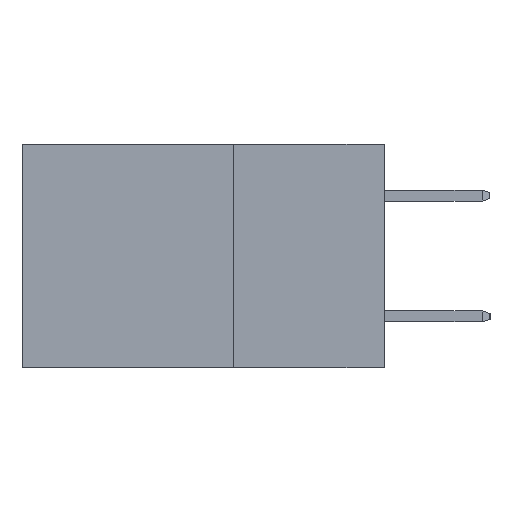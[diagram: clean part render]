
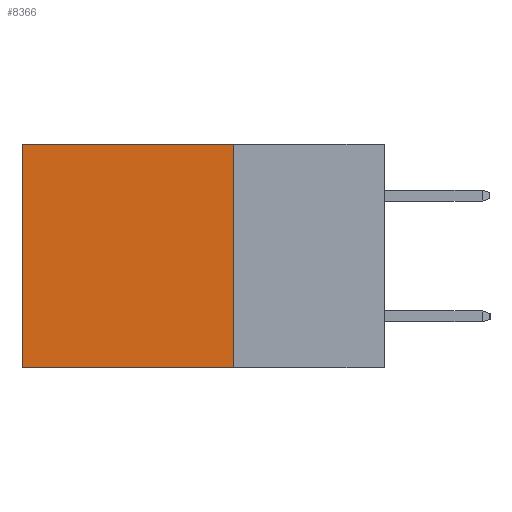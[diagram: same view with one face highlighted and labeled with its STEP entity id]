
A CAD part, left-side view. The second image highlights one B-rep face of the part: STEP entity #8366.
In plain terms, the highlighted planar face has unit normal (-1, 0, 0).
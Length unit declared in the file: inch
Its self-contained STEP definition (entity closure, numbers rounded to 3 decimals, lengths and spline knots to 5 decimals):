
#204 = DIRECTION ( 'NONE',  ( 0., 1., 0. ) ) ;
#207 = CARTESIAN_POINT ( 'NONE',  ( 0.2615, 0.25, -0.37 ) ) ;
#211 = ORIENTED_EDGE ( 'NONE', *, *, #9571, .F. ) ;
#491 = ORIENTED_EDGE ( 'NONE', *, *, #6618, .T. ) ;
#610 = DIRECTION ( 'NONE',  ( 0., 0., -1. ) ) ;
#867 = AXIS2_PLACEMENT_3D ( 'NONE', #12102, #6731, #6698 ) ;
#1124 = FACE_OUTER_BOUND ( 'NONE', #7912, .T. ) ;
#1411 = LINE ( 'NONE', #207, #10693 ) ;
#1693 = CARTESIAN_POINT ( 'NONE',  ( 0.2615, 0.25, -0.37 ) ) ;
#1770 = VECTOR ( 'NONE', #4200, 39.37008 ) ;
#1821 = ORIENTED_EDGE ( 'NONE', *, *, #10764, .F. ) ;
#2172 = VERTEX_POINT ( 'NONE', #12283 ) ;
#2630 = ORIENTED_EDGE ( 'NONE', *, *, #12845, .T. ) ;
#3161 = LINE ( 'NONE', #4445, #11284 ) ;
#3537 = VERTEX_POINT ( 'NONE', #5092 ) ;
#4200 = DIRECTION ( 'NONE',  ( 0., 0., -1. ) ) ;
#4445 = CARTESIAN_POINT ( 'NONE',  ( 0.2615, 0.25, 0. ) ) ;
#4867 = LINE ( 'NONE', #7555, #1770 ) ;
#5092 = CARTESIAN_POINT ( 'NONE',  ( 0.2615, 0.25, 0. ) ) ;
#5323 = CARTESIAN_POINT ( 'NONE',  ( 0.2615, 0.25, -0.37 ) ) ;
#5621 = CARTESIAN_POINT ( 'NONE',  ( 0.2615, 0.6, -0.37 ) ) ;
#5635 = DIRECTION ( 'NONE',  ( 0., 1., 0. ) ) ;
#5940 = VERTEX_POINT ( 'NONE', #5621 ) ;
#6618 = EDGE_CURVE ( 'NONE', #3537, #2172, #3161, .T. ) ;
#6698 = DIRECTION ( 'NONE',  ( 0., 0., -1. ) ) ;
#6731 = DIRECTION ( 'NONE',  ( 1., 0., 0. ) ) ;
#7555 = CARTESIAN_POINT ( 'NONE',  ( 0.2615, 0.6, -0.37 ) ) ;
#7912 = EDGE_LOOP ( 'NONE', ( #2630, #1821, #211, #491 ) ) ;
#8366 = ADVANCED_FACE ( 'NONE', ( #1124 ), #13477, .F. ) ;
#8513 = VECTOR ( 'NONE', #610, 39.37008 ) ;
#9571 = EDGE_CURVE ( 'NONE', #3537, #10927, #11369, .T. ) ;
#10693 = VECTOR ( 'NONE', #204, 39.37008 ) ;
#10764 = EDGE_CURVE ( 'NONE', #10927, #5940, #1411, .T. ) ;
#10927 = VERTEX_POINT ( 'NONE', #5323 ) ;
#11284 = VECTOR ( 'NONE', #5635, 39.37008 ) ;
#11369 = LINE ( 'NONE', #1693, #8513 ) ;
#12102 = CARTESIAN_POINT ( 'NONE',  ( 0.2615, 0.25, -0.37 ) ) ;
#12283 = CARTESIAN_POINT ( 'NONE',  ( 0.2615, 0.6, 0. ) ) ;
#12845 = EDGE_CURVE ( 'NONE', #2172, #5940, #4867, .T. ) ;
#13477 = PLANE ( 'NONE',  #867 ) ;
